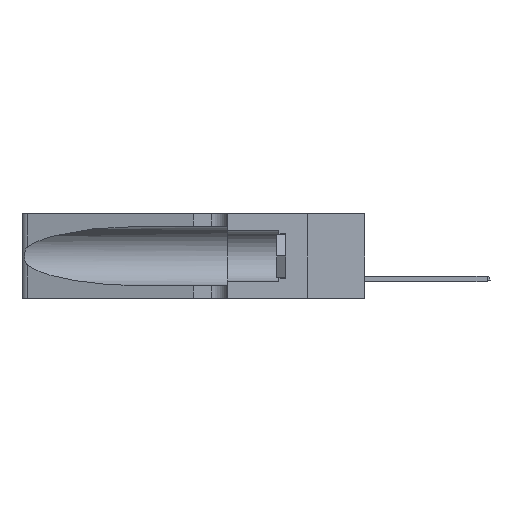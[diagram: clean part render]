
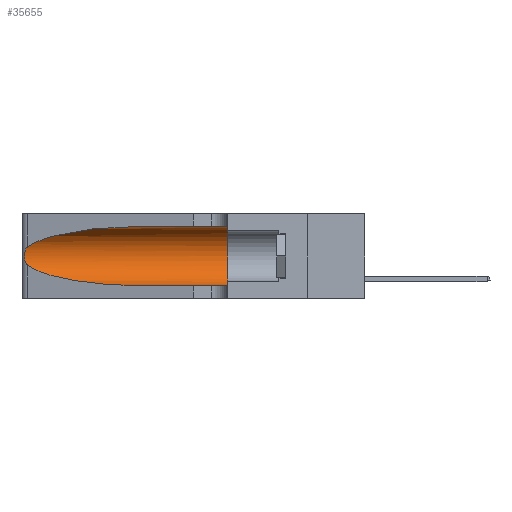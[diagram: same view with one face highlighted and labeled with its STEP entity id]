
A CAD part, left-side view. The second image highlights one B-rep face of the part: STEP entity #35655.
In plain terms, the highlighted cylindrical face has radius 3.308 mm (diameter 6.617 mm), a partial arc.
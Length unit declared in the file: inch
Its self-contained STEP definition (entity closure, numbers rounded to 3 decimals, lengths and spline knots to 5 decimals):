
#220 = B_SPLINE_CURVE_WITH_KNOTS ( 'NONE', 3,
 ( #36266, #26917, #12139, #446, #33019, #15151, #21416, #3430, #24406, #704, #25062, #16174, #28051, #27639 ),
 .UNSPECIFIED., .F., .F.,
 ( 4, 2, 2, 2, 2, 2, 4 ),
 ( 0., 0.00027, 0.00053, 0.00107, 0.0016, 0.00187, 0.00214 ),
 .UNSPECIFIED. ) ;
#446 = CARTESIAN_POINT ( 'NONE',  ( 0.25787, 1.23484, 0.2124 ) ) ;
#602 = FACE_OUTER_BOUND ( 'NONE', #5161, .T. ) ;
#704 = CARTESIAN_POINT ( 'NONE',  ( 0.25856, 1.23593, 0.16098 ) ) ;
#740 = CARTESIAN_POINT ( 'NONE',  ( 0.1305, 0.35, 0.05475 ) ) ;
#1170 = ORIENTED_EDGE ( 'NONE', *, *, #24899, .F. ) ;
#1425 = EDGE_CURVE ( 'NONE', #28081, #11253, #32432, .T. ) ;
#3430 = CARTESIAN_POINT ( 'NONE',  ( 0.26075, 1.23896, 0.178 ) ) ;
#3520 = CARTESIAN_POINT ( 'NONE',  ( 0.1305, 1.61858, 0.31525 ) ) ;
#3664 = CARTESIAN_POINT ( 'NONE',  ( 0.1305, 1.61858, 0.185 ) ) ;
#4236 = DIRECTION ( 'NONE',  ( 0., 1., 0. ) ) ;
#4848 =( BOUNDED_CURVE ( )  B_SPLINE_CURVE ( 3, ( #25441, #31839, #25983, #7910 ),
 .UNSPECIFIED., .F., .T. ) 
 B_SPLINE_CURVE_WITH_KNOTS ( ( 4, 4 ),
 ( 1.5708, 2.84003 ),
 .UNSPECIFIED. ) 
 CURVE ( )  GEOMETRIC_REPRESENTATION_ITEM ( )  RATIONAL_B_SPLINE_CURVE ( ( 1., 0.87, 0.87, 1. ) ) 
 REPRESENTATION_ITEM ( '' )  );
#4911 = CARTESIAN_POINT ( 'NONE',  ( 0.1305, 0.72297, 0.31525 ) ) ;
#4915 = CARTESIAN_POINT ( 'NONE',  ( 0.25487, 1.22718, 0.22369 ) ) ;
#5161 = EDGE_LOOP ( 'NONE', ( #34815, #38626, #21298, #30922, #1170, #36894 ) ) ;
#5329 = CARTESIAN_POINT ( 'NONE',  ( 0.25487, 1.22718, 0.14631 ) ) ;
#5594 = CARTESIAN_POINT ( 'NONE',  ( 0.18966, 0.96281, 0.05475 ) ) ;
#5718 = CARTESIAN_POINT ( 'NONE',  ( 0.1305, 0.72297, 0.05475 ) ) ;
#7248 = DIRECTION ( 'NONE',  ( 0., 0., 1. ) ) ;
#7910 = CARTESIAN_POINT ( 'NONE',  ( 0.25487, 1.22718, 0.22369 ) ) ;
#8709 = DIRECTION ( 'NONE',  ( 0., 0., -1. ) ) ;
#8815 = VECTOR ( 'NONE', #21790, 39.37008 ) ;
#11253 = VERTEX_POINT ( 'NONE', #35529 ) ;
#12139 = CARTESIAN_POINT ( 'NONE',  ( 0.25639, 1.23184, 0.21858 ) ) ;
#12897 = EDGE_CURVE ( 'NONE', #30416, #15886, #36362, .T. ) ;
#13527 = VERTEX_POINT ( 'NONE', #4915 ) ;
#15151 = CARTESIAN_POINT ( 'NONE',  ( 0.26018, 1.23835, 0.19895 ) ) ;
#15886 = VERTEX_POINT ( 'NONE', #27803 ) ;
#16174 = CARTESIAN_POINT ( 'NONE',  ( 0.25639, 1.23186, 0.15144 ) ) ;
#17790 = AXIS2_PLACEMENT_3D ( 'NONE', #30882, #4236, #7248 ) ;
#20020 = VECTOR ( 'NONE', #23587, 39.37008 ) ;
#21298 = ORIENTED_EDGE ( 'NONE', *, *, #1425, .T. ) ;
#21416 = CARTESIAN_POINT ( 'NONE',  ( 0.26075, 1.23896, 0.19203 ) ) ;
#21790 = DIRECTION ( 'NONE',  ( 0., -1., 0. ) ) ;
#22867 = EDGE_CURVE ( 'NONE', #13527, #28081, #220, .T. ) ;
#23587 = DIRECTION ( 'NONE',  ( 0., -1., 0. ) ) ;
#24406 = CARTESIAN_POINT ( 'NONE',  ( 0.26017, 1.23833, 0.17102 ) ) ;
#24632 = DIRECTION ( 'NONE',  ( 0., -1., 0. ) ) ;
#24899 = EDGE_CURVE ( 'NONE', #15886, #35237, #33155, .T. ) ;
#25062 = CARTESIAN_POINT ( 'NONE',  ( 0.25789, 1.23486, 0.15765 ) ) ;
#25441 = CARTESIAN_POINT ( 'NONE',  ( 0.1305, 0.72297, 0.31525 ) ) ;
#25533 = AXIS2_PLACEMENT_3D ( 'NONE', #3664, #24632, #8709 ) ;
#25983 = CARTESIAN_POINT ( 'NONE',  ( 0.2373, 1.15595, 0.28018 ) ) ;
#26402 = CARTESIAN_POINT ( 'NONE',  ( 0.1305, 1.61858, 0.05475 ) ) ;
#26917 = CARTESIAN_POINT ( 'NONE',  ( 0.25555, 1.22994, 0.2215 ) ) ;
#27639 = CARTESIAN_POINT ( 'NONE',  ( 0.25487, 1.22718, 0.14631 ) ) ;
#27803 = CARTESIAN_POINT ( 'NONE',  ( 0.1305, 0.35, 0.31525 ) ) ;
#28051 = CARTESIAN_POINT ( 'NONE',  ( 0.25555, 1.22993, 0.14849 ) ) ;
#28081 = VERTEX_POINT ( 'NONE', #36976 ) ;
#29526 = CARTESIAN_POINT ( 'NONE',  ( 0.2373, 1.15595, 0.08982 ) ) ;
#30378 = EDGE_CURVE ( 'NONE', #30416, #13527, #4848, .T. ) ;
#30416 = VERTEX_POINT ( 'NONE', #4911 ) ;
#30882 = CARTESIAN_POINT ( 'NONE',  ( 0.1305, 0.35, 0.185 ) ) ;
#30922 = ORIENTED_EDGE ( 'NONE', *, *, #34958, .T. ) ;
#31839 = CARTESIAN_POINT ( 'NONE',  ( 0.18966, 0.96281, 0.31525 ) ) ;
#32432 =( BOUNDED_CURVE ( )  B_SPLINE_CURVE ( 3, ( #5329, #29526, #5594, #5718 ),
 .UNSPECIFIED., .F., .F. ) 
 B_SPLINE_CURVE_WITH_KNOTS ( ( 4, 4 ),
 ( 3.44316, 4.71239 ),
 .UNSPECIFIED. ) 
 CURVE ( )  GEOMETRIC_REPRESENTATION_ITEM ( )  RATIONAL_B_SPLINE_CURVE ( ( 1., 0.87, 0.87, 1. ) ) 
 REPRESENTATION_ITEM ( '' )  );
#33019 = CARTESIAN_POINT ( 'NONE',  ( 0.25854, 1.2359, 0.20912 ) ) ;
#33155 = CIRCLE ( 'NONE', #17790, 0.13025 ) ;
#34815 = ORIENTED_EDGE ( 'NONE', *, *, #30378, .T. ) ;
#34958 = EDGE_CURVE ( 'NONE', #11253, #35237, #38680, .T. ) ;
#35237 = VERTEX_POINT ( 'NONE', #740 ) ;
#35529 = CARTESIAN_POINT ( 'NONE',  ( 0.1305, 0.72297, 0.05475 ) ) ;
#35655 = ADVANCED_FACE ( 'NONE', ( #602 ), #38610, .F. ) ;
#36266 = CARTESIAN_POINT ( 'NONE',  ( 0.25487, 1.22718, 0.22369 ) ) ;
#36362 = LINE ( 'NONE', #3520, #8815 ) ;
#36894 = ORIENTED_EDGE ( 'NONE', *, *, #12897, .F. ) ;
#36976 = CARTESIAN_POINT ( 'NONE',  ( 0.25487, 1.22718, 0.14631 ) ) ;
#38610 = CYLINDRICAL_SURFACE ( 'NONE', #25533, 0.13025 ) ;
#38626 = ORIENTED_EDGE ( 'NONE', *, *, #22867, .T. ) ;
#38680 = LINE ( 'NONE', #26402, #20020 ) ;
